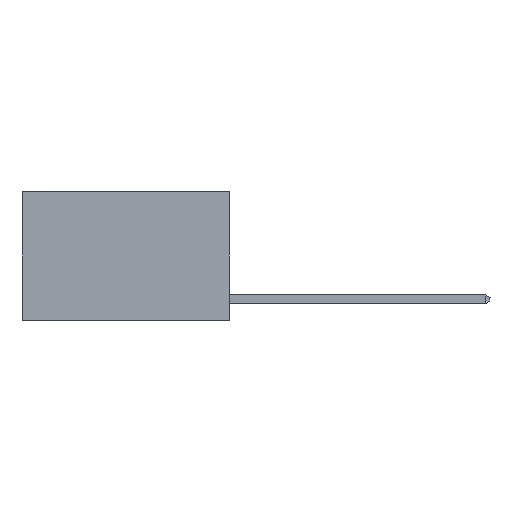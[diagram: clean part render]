
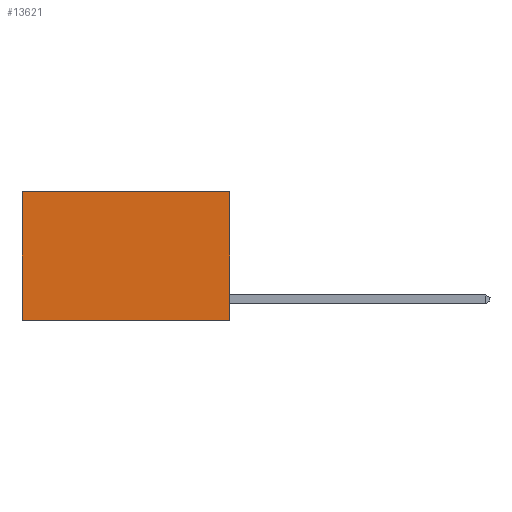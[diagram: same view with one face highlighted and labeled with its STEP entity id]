
A CAD part, left-side view. The second image highlights one B-rep face of the part: STEP entity #13621.
In plain terms, the highlighted planar face has unit normal (-1, 0, 0).
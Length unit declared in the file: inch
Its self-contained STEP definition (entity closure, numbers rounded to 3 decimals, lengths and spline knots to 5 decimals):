
#368 = EDGE_CURVE ( 'NONE', #17625, #11719, #14053, .T. ) ;
#510 = VERTEX_POINT ( 'NONE', #11363 ) ;
#599 = ORIENTED_EDGE ( 'NONE', *, *, #6798, .T. ) ;
#842 = FACE_OUTER_BOUND ( 'NONE', #17891, .T. ) ;
#2457 = VERTEX_POINT ( 'NONE', #8491 ) ;
#4062 = EDGE_CURVE ( 'NONE', #11719, #2457, #7805, .T. ) ;
#4538 = VECTOR ( 'NONE', #5263, 39.37008 ) ;
#4548 = CARTESIAN_POINT ( 'NONE',  ( 0.2625, 0., 0. ) ) ;
#4558 = DIRECTION ( 'NONE',  ( 0., 0., -1. ) ) ;
#4613 = LINE ( 'NONE', #15125, #15486 ) ;
#5263 = DIRECTION ( 'NONE',  ( 0., 0., -1. ) ) ;
#6798 = EDGE_CURVE ( 'NONE', #510, #2457, #4613, .T. ) ;
#7805 = LINE ( 'NONE', #21648, #21461 ) ;
#8491 = CARTESIAN_POINT ( 'NONE',  ( 0.2625, 0.6, -0.37 ) ) ;
#9476 = CARTESIAN_POINT ( 'NONE',  ( 0.2625, 0., 0. ) ) ;
#10782 = CARTESIAN_POINT ( 'NONE',  ( 0.2625, 0., -0.37 ) ) ;
#11363 = CARTESIAN_POINT ( 'NONE',  ( 0.2625, 0.6, 0. ) ) ;
#11429 = LINE ( 'NONE', #13612, #16790 ) ;
#11644 = DIRECTION ( 'NONE',  ( 0., 0., -1. ) ) ;
#11719 = VERTEX_POINT ( 'NONE', #10782 ) ;
#12813 = AXIS2_PLACEMENT_3D ( 'NONE', #9476, #20082, #4558 ) ;
#12993 = PLANE ( 'NONE',  #12813 ) ;
#13612 = CARTESIAN_POINT ( 'NONE',  ( 0.2625, 0., 0. ) ) ;
#13621 = ADVANCED_FACE ( 'NONE', ( #842 ), #12993, .F. ) ;
#14053 = LINE ( 'NONE', #15567, #4538 ) ;
#15125 = CARTESIAN_POINT ( 'NONE',  ( 0.2625, 0.6, 0. ) ) ;
#15486 = VECTOR ( 'NONE', #11644, 39.37008 ) ;
#15567 = CARTESIAN_POINT ( 'NONE',  ( 0.2625, 0., 0. ) ) ;
#16790 = VECTOR ( 'NONE', #22021, 39.37008 ) ;
#17625 = VERTEX_POINT ( 'NONE', #4548 ) ;
#17891 = EDGE_LOOP ( 'NONE', ( #599, #18002, #20938, #20276 ) ) ;
#18002 = ORIENTED_EDGE ( 'NONE', *, *, #4062, .F. ) ;
#20082 = DIRECTION ( 'NONE',  ( 1., 0., 0. ) ) ;
#20276 = ORIENTED_EDGE ( 'NONE', *, *, #22890, .T. ) ;
#20938 = ORIENTED_EDGE ( 'NONE', *, *, #368, .F. ) ;
#21461 = VECTOR ( 'NONE', #21769, 39.37008 ) ;
#21648 = CARTESIAN_POINT ( 'NONE',  ( 0.2625, 0., -0.37 ) ) ;
#21769 = DIRECTION ( 'NONE',  ( 0., 1., 0. ) ) ;
#22021 = DIRECTION ( 'NONE',  ( 0., 1., 0. ) ) ;
#22890 = EDGE_CURVE ( 'NONE', #17625, #510, #11429, .T. ) ;
